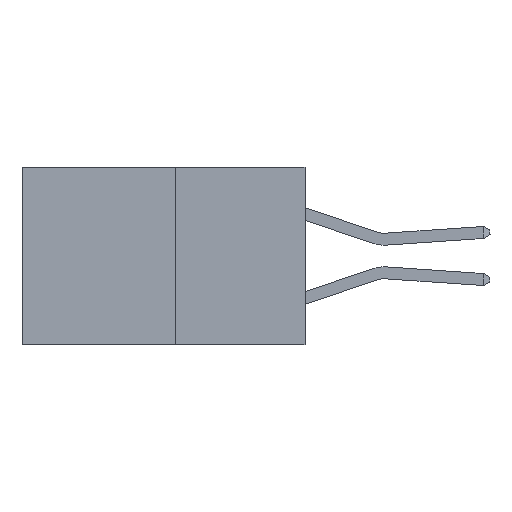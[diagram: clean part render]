
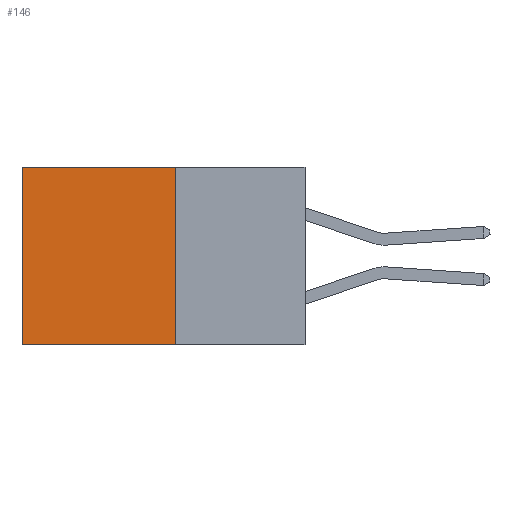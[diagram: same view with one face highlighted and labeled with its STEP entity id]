
A CAD part, left-side view. The second image highlights one B-rep face of the part: STEP entity #146.
In plain terms, the highlighted planar face has unit normal (-1, 0, 0).
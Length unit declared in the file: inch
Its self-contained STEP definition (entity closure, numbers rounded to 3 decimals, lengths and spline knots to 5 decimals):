
#146 = ADVANCED_FACE ( 'NONE', ( #5724 ), #7413, .F. ) ;
#332 = CARTESIAN_POINT ( 'NONE',  ( 0.277, 0.27, -0.37 ) ) ;
#376 = DIRECTION ( 'NONE',  ( 0., 0., -1. ) ) ;
#758 = EDGE_CURVE ( 'NONE', #6411, #7596, #6777, .T. ) ;
#1027 = CARTESIAN_POINT ( 'NONE',  ( 0.277, 0.27, 0. ) ) ;
#1355 = CARTESIAN_POINT ( 'NONE',  ( 0.277, 0.59, -0.37 ) ) ;
#1537 = EDGE_CURVE ( 'NONE', #7596, #5213, #7443, .T. ) ;
#1634 = DIRECTION ( 'NONE',  ( 1., 0., 0. ) ) ;
#1780 = EDGE_CURVE ( 'NONE', #6411, #2116, #5347, .T. ) ;
#2116 = VERTEX_POINT ( 'NONE', #4451 ) ;
#2790 = VECTOR ( 'NONE', #376, 39.37008 ) ;
#2932 = EDGE_CURVE ( 'NONE', #2116, #5213, #6028, .T. ) ;
#2962 = ORIENTED_EDGE ( 'NONE', *, *, #2932, .T. ) ;
#3059 = CARTESIAN_POINT ( 'NONE',  ( 0.277, 0.27, -0.37 ) ) ;
#3086 = EDGE_LOOP ( 'NONE', ( #2962, #5423, #5902, #8740 ) ) ;
#3781 = VECTOR ( 'NONE', #4369, 39.37008 ) ;
#4061 = VECTOR ( 'NONE', #8321, 39.37008 ) ;
#4369 = DIRECTION ( 'NONE',  ( 0., 0., -1. ) ) ;
#4451 = CARTESIAN_POINT ( 'NONE',  ( 0.277, 0.59, 0. ) ) ;
#4709 = CARTESIAN_POINT ( 'NONE',  ( 0.277, 0.27, 0. ) ) ;
#4921 = CARTESIAN_POINT ( 'NONE',  ( 0.277, 0.27, -0.37 ) ) ;
#5213 = VERTEX_POINT ( 'NONE', #1355 ) ;
#5347 = LINE ( 'NONE', #4709, #4061 ) ;
#5423 = ORIENTED_EDGE ( 'NONE', *, *, #1537, .F. ) ;
#5724 = FACE_OUTER_BOUND ( 'NONE', #3086, .T. ) ;
#5858 = DIRECTION ( 'NONE',  ( 0., 0., -1. ) ) ;
#5894 = AXIS2_PLACEMENT_3D ( 'NONE', #332, #1634, #5858 ) ;
#5902 = ORIENTED_EDGE ( 'NONE', *, *, #758, .F. ) ;
#6028 = LINE ( 'NONE', #6797, #3781 ) ;
#6153 = CARTESIAN_POINT ( 'NONE',  ( 0.277, 0.27, -0.37 ) ) ;
#6411 = VERTEX_POINT ( 'NONE', #1027 ) ;
#6777 = LINE ( 'NONE', #4921, #2790 ) ;
#6797 = CARTESIAN_POINT ( 'NONE',  ( 0.277, 0.59, -0.37 ) ) ;
#7413 = PLANE ( 'NONE',  #5894 ) ;
#7443 = LINE ( 'NONE', #3059, #9564 ) ;
#7596 = VERTEX_POINT ( 'NONE', #6153 ) ;
#8321 = DIRECTION ( 'NONE',  ( 0., 1., 0. ) ) ;
#8740 = ORIENTED_EDGE ( 'NONE', *, *, #1780, .T. ) ;
#9242 = DIRECTION ( 'NONE',  ( 0., 1., 0. ) ) ;
#9564 = VECTOR ( 'NONE', #9242, 39.37008 ) ;
